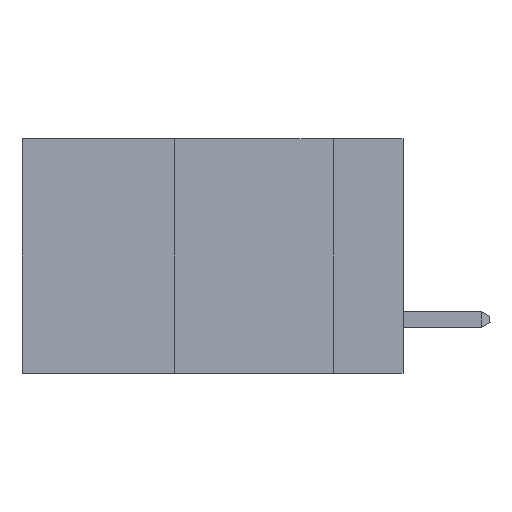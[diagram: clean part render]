
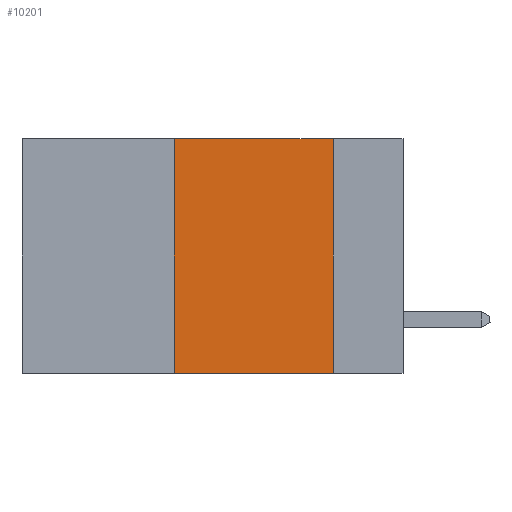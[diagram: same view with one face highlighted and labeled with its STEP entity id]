
A CAD part, left-side view. The second image highlights one B-rep face of the part: STEP entity #10201.
In plain terms, the highlighted planar face has unit normal (-1, 0, 0).
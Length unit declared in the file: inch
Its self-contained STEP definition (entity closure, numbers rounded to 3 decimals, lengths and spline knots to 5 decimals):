
#309 = ORIENTED_EDGE ( 'NONE', *, *, #23762, .T. ) ;
#2261 = EDGE_LOOP ( 'NONE', ( #5512, #6540, #18556, #309 ) ) ;
#3568 = VECTOR ( 'NONE', #23789, 39.37008 ) ;
#4568 = DIRECTION ( 'NONE',  ( 0., -1., 0. ) ) ;
#5143 = VECTOR ( 'NONE', #20711, 39.37008 ) ;
#5512 = ORIENTED_EDGE ( 'NONE', *, *, #22550, .F. ) ;
#6150 = CARTESIAN_POINT ( 'NONE',  ( 0., 0.36, 0. ) ) ;
#6254 = VERTEX_POINT ( 'NONE', #9753 ) ;
#6540 = ORIENTED_EDGE ( 'NONE', *, *, #16608, .F. ) ;
#6823 = EDGE_CURVE ( 'NONE', #20918, #23565, #24597, .T. ) ;
#8063 = CARTESIAN_POINT ( 'NONE',  ( 0., 0.6, 0. ) ) ;
#9163 = DIRECTION ( 'NONE',  ( 0., -1., 0. ) ) ;
#9600 = CARTESIAN_POINT ( 'NONE',  ( 0., 0.36, -0.37 ) ) ;
#9753 = CARTESIAN_POINT ( 'NONE',  ( 0., 0.11, 0. ) ) ;
#10071 = DIRECTION ( 'NONE',  ( 0., 0., -1. ) ) ;
#10197 = FACE_OUTER_BOUND ( 'NONE', #2261, .T. ) ;
#10201 = ADVANCED_FACE ( 'NONE', ( #10197 ), #19902, .F. ) ;
#11041 = LINE ( 'NONE', #13786, #20924 ) ;
#13404 = LINE ( 'NONE', #24859, #24850 ) ;
#13786 = CARTESIAN_POINT ( 'NONE',  ( 0., 0.6, 0. ) ) ;
#13845 = CARTESIAN_POINT ( 'NONE',  ( 0., 0.36, 0. ) ) ;
#15872 = AXIS2_PLACEMENT_3D ( 'NONE', #8063, #21871, #10071 ) ;
#16608 = EDGE_CURVE ( 'NONE', #23565, #6254, #11041, .T. ) ;
#17063 = VERTEX_POINT ( 'NONE', #21778 ) ;
#18556 = ORIENTED_EDGE ( 'NONE', *, *, #6823, .F. ) ;
#19902 = PLANE ( 'NONE',  #15872 ) ;
#20711 = DIRECTION ( 'NONE',  ( 0., 0., -1. ) ) ;
#20918 = VERTEX_POINT ( 'NONE', #9600 ) ;
#20924 = VECTOR ( 'NONE', #4568, 39.37008 ) ;
#21778 = CARTESIAN_POINT ( 'NONE',  ( 0., 0.11, -0.37 ) ) ;
#21871 = DIRECTION ( 'NONE',  ( 1., 0., 0. ) ) ;
#22171 = CARTESIAN_POINT ( 'NONE',  ( 0., 0.11, 0. ) ) ;
#22550 = EDGE_CURVE ( 'NONE', #6254, #17063, #24955, .T. ) ;
#23565 = VERTEX_POINT ( 'NONE', #6150 ) ;
#23762 = EDGE_CURVE ( 'NONE', #20918, #17063, #13404, .T. ) ;
#23789 = DIRECTION ( 'NONE',  ( 0., 0., 1. ) ) ;
#24597 = LINE ( 'NONE', #13845, #3568 ) ;
#24850 = VECTOR ( 'NONE', #9163, 39.37008 ) ;
#24859 = CARTESIAN_POINT ( 'NONE',  ( 0., 0.6, -0.37 ) ) ;
#24955 = LINE ( 'NONE', #22171, #5143 ) ;
